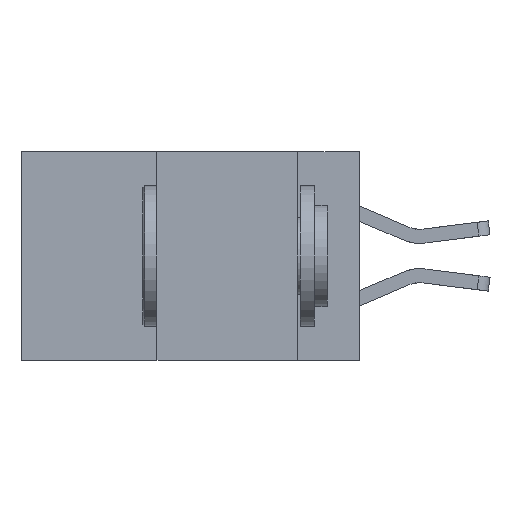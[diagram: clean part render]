
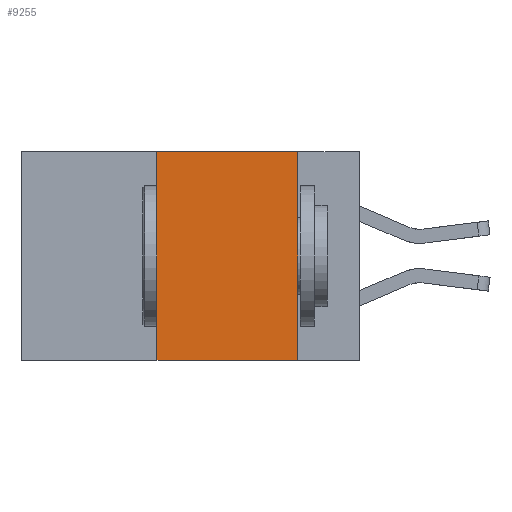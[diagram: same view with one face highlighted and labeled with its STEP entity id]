
A CAD part, left-side view. The second image highlights one B-rep face of the part: STEP entity #9255.
In plain terms, the highlighted planar face has unit normal (-1, 0, 0).
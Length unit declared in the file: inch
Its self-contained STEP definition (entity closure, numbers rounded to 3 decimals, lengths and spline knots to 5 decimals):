
#177 = VERTEX_POINT ( 'NONE', #1131 ) ;
#214 = LINE ( 'NONE', #618, #1345 ) ;
#502 = ORIENTED_EDGE ( 'NONE', *, *, #8586, .T. ) ;
#618 = CARTESIAN_POINT ( 'NONE',  ( 0., 0.6, 0. ) ) ;
#661 = FACE_OUTER_BOUND ( 'NONE', #8208, .T. ) ;
#735 = CARTESIAN_POINT ( 'NONE',  ( 0., 0.11, 0. ) ) ;
#1115 = CARTESIAN_POINT ( 'NONE',  ( 0., 0.6, -0.37 ) ) ;
#1131 = CARTESIAN_POINT ( 'NONE',  ( 0., 0.36, -0.37 ) ) ;
#1345 = VECTOR ( 'NONE', #10122, 39.37008 ) ;
#1993 = ORIENTED_EDGE ( 'NONE', *, *, #10316, .F. ) ;
#3092 = CARTESIAN_POINT ( 'NONE',  ( 0., 0.11, 0. ) ) ;
#4019 = VERTEX_POINT ( 'NONE', #3092 ) ;
#4878 = VECTOR ( 'NONE', #9303, 39.37008 ) ;
#5538 = EDGE_CURVE ( 'NONE', #5839, #4019, #214, .T. ) ;
#5599 = VECTOR ( 'NONE', #10345, 39.37008 ) ;
#5839 = VERTEX_POINT ( 'NONE', #9686 ) ;
#6581 = LINE ( 'NONE', #735, #12099 ) ;
#6705 = DIRECTION ( 'NONE',  ( 0., 0., -1. ) ) ;
#7182 = EDGE_CURVE ( 'NONE', #4019, #13367, #6581, .T. ) ;
#7212 = DIRECTION ( 'NONE',  ( 1., 0., 0. ) ) ;
#7854 = ORIENTED_EDGE ( 'NONE', *, *, #7182, .F. ) ;
#8208 = EDGE_LOOP ( 'NONE', ( #7854, #8681, #1993, #502 ) ) ;
#8357 = CARTESIAN_POINT ( 'NONE',  ( 0., 0.11, -0.37 ) ) ;
#8454 = DIRECTION ( 'NONE',  ( 0., 0., -1. ) ) ;
#8586 = EDGE_CURVE ( 'NONE', #177, #13367, #12243, .T. ) ;
#8681 = ORIENTED_EDGE ( 'NONE', *, *, #5538, .F. ) ;
#9255 = ADVANCED_FACE ( 'NONE', ( #661 ), #14332, .F. ) ;
#9303 = DIRECTION ( 'NONE',  ( 0., -1., 0. ) ) ;
#9686 = CARTESIAN_POINT ( 'NONE',  ( 0., 0.36, 0. ) ) ;
#9932 = AXIS2_PLACEMENT_3D ( 'NONE', #14284, #7212, #8454 ) ;
#10122 = DIRECTION ( 'NONE',  ( 0., -1., 0. ) ) ;
#10316 = EDGE_CURVE ( 'NONE', #177, #5839, #14625, .T. ) ;
#10345 = DIRECTION ( 'NONE',  ( 0., 0., 1. ) ) ;
#12099 = VECTOR ( 'NONE', #6705, 39.37008 ) ;
#12243 = LINE ( 'NONE', #1115, #4878 ) ;
#13367 = VERTEX_POINT ( 'NONE', #8357 ) ;
#13845 = CARTESIAN_POINT ( 'NONE',  ( 0., 0.36, 0. ) ) ;
#14284 = CARTESIAN_POINT ( 'NONE',  ( 0., 0.6, 0. ) ) ;
#14332 = PLANE ( 'NONE',  #9932 ) ;
#14625 = LINE ( 'NONE', #13845, #5599 ) ;
